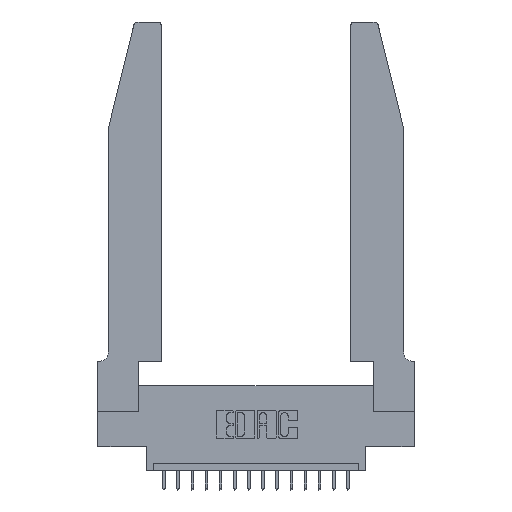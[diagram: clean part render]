
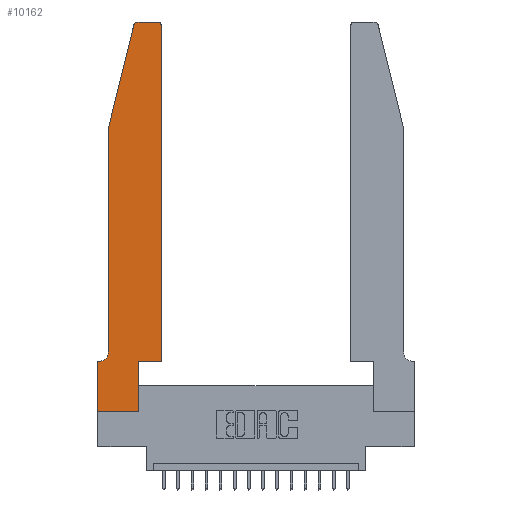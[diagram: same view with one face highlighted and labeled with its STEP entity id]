
A CAD part, top view. The second image highlights one B-rep face of the part: STEP entity #10162.
In plain terms, the highlighted planar face has unit normal (0, 0, 1).
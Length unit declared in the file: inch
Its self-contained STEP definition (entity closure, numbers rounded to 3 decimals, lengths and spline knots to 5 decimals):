
#179 = DIRECTION ( 'NONE',  ( 0., -1., 0. ) ) ;
#276 = EDGE_CURVE ( 'NONE', #15528, #753, #18520, .T. ) ;
#481 = DIRECTION ( 'NONE',  ( 1., 0., 0. ) ) ;
#716 = LINE ( 'NONE', #3756, #17238 ) ;
#753 = VERTEX_POINT ( 'NONE', #8095 ) ;
#1276 = CIRCLE ( 'NONE', #10348, 0.07 ) ;
#1418 = LINE ( 'NONE', #9024, #13395 ) ;
#1713 = VERTEX_POINT ( 'NONE', #18773 ) ;
#1873 = ORIENTED_EDGE ( 'NONE', *, *, #7005, .T. ) ;
#2048 = DIRECTION ( 'NONE',  ( 1., 0., 0. ) ) ;
#2084 = ORIENTED_EDGE ( 'NONE', *, *, #11575, .T. ) ;
#2132 = CARTESIAN_POINT ( 'NONE',  ( 0.4505, 0.35, 0.37 ) ) ;
#2269 = ORIENTED_EDGE ( 'NONE', *, *, #15552, .T. ) ;
#2403 = CARTESIAN_POINT ( 'NONE',  ( 0., 0.35, 0.37 ) ) ;
#2612 = EDGE_CURVE ( 'NONE', #7408, #15528, #11986, .T. ) ;
#2726 = LINE ( 'NONE', #2132, #7261 ) ;
#3155 = VECTOR ( 'NONE', #179, 39.37008 ) ;
#3355 = ORIENTED_EDGE ( 'NONE', *, *, #2612, .T. ) ;
#3377 = ORIENTED_EDGE ( 'NONE', *, *, #5155, .T. ) ;
#3412 = CARTESIAN_POINT ( 'NONE',  ( 0., 0., 0.37 ) ) ;
#3501 = VERTEX_POINT ( 'NONE', #7118 ) ;
#3566 = VECTOR ( 'NONE', #12857, 39.37008 ) ;
#3584 = PLANE ( 'NONE',  #14703 ) ;
#3756 = CARTESIAN_POINT ( 'NONE',  ( 0.0755, 2., 0.37 ) ) ;
#3758 = EDGE_CURVE ( 'NONE', #17499, #9092, #2726, .T. ) ;
#4745 = ORIENTED_EDGE ( 'NONE', *, *, #13297, .T. ) ;
#5133 = CARTESIAN_POINT ( 'NONE',  ( 0.2865, 0.35, 0.37 ) ) ;
#5155 = EDGE_CURVE ( 'NONE', #9092, #3501, #14441, .T. ) ;
#5293 = EDGE_CURVE ( 'NONE', #18282, #9228, #18702, .T. ) ;
#5518 = LINE ( 'NONE', #11480, #9516 ) ;
#5533 = CARTESIAN_POINT ( 'NONE',  ( 0.4505, 0.35, 0.37 ) ) ;
#5804 = CARTESIAN_POINT ( 'NONE',  ( 0.0755, 0.42, 0.37 ) ) ;
#6285 = AXIS2_PLACEMENT_3D ( 'NONE', #13538, #7651, #9419 ) ;
#6361 = CARTESIAN_POINT ( 'NONE',  ( 0.0055, 0.42, 0.37 ) ) ;
#6548 = DIRECTION ( 'NONE',  ( 0., 0., -1. ) ) ;
#6623 = CARTESIAN_POINT ( 'NONE',  ( 0.25487, 2.72718, 0.37 ) ) ;
#6675 = CARTESIAN_POINT ( 'NONE',  ( 0.0055, 0.35, 0.37 ) ) ;
#6748 = ORIENTED_EDGE ( 'NONE', *, *, #8304, .T. ) ;
#6881 = CARTESIAN_POINT ( 'NONE',  ( 0.0755, 2., 0.37 ) ) ;
#6970 = VECTOR ( 'NONE', #16101, 39.37008 ) ;
#7005 = EDGE_CURVE ( 'NONE', #10251, #7408, #1418, .T. ) ;
#7050 = DIRECTION ( 'NONE',  ( -1., 0., 0. ) ) ;
#7052 = VERTEX_POINT ( 'NONE', #5804 ) ;
#7118 = CARTESIAN_POINT ( 'NONE',  ( 0.4505, 2.72, 0.37 ) ) ;
#7261 = VECTOR ( 'NONE', #2048, 39.37008 ) ;
#7308 = CARTESIAN_POINT ( 'NONE',  ( 0.4505, 0.35, 0.37 ) ) ;
#7408 = VERTEX_POINT ( 'NONE', #13097 ) ;
#7572 = DIRECTION ( 'NONE',  ( 0., 0., 1. ) ) ;
#7651 = DIRECTION ( 'NONE',  ( 0., 0., 1. ) ) ;
#7834 = LINE ( 'NONE', #11001, #16626 ) ;
#8095 = CARTESIAN_POINT ( 'NONE',  ( 0.2865, 0., 0.37 ) ) ;
#8236 = ORIENTED_EDGE ( 'NONE', *, *, #13057, .T. ) ;
#8304 = EDGE_CURVE ( 'NONE', #7052, #10251, #1276, .T. ) ;
#8344 = VECTOR ( 'NONE', #481, 39.37008 ) ;
#9024 = CARTESIAN_POINT ( 'NONE',  ( 0.0755, 0.35, 0.37 ) ) ;
#9092 = VERTEX_POINT ( 'NONE', #5533 ) ;
#9107 = CARTESIAN_POINT ( 'NONE',  ( 0.0755, 2., 0.37 ) ) ;
#9228 = VERTEX_POINT ( 'NONE', #9107 ) ;
#9369 = CIRCLE ( 'NONE', #12194, 0.03 ) ;
#9419 = DIRECTION ( 'NONE',  ( 1., 0., 0. ) ) ;
#9516 = VECTOR ( 'NONE', #7050, 39.37008 ) ;
#9630 = DIRECTION ( 'NONE',  ( 0., 0., 1. ) ) ;
#9719 = DIRECTION ( 'NONE',  ( 0., -1., 0. ) ) ;
#9969 = VERTEX_POINT ( 'NONE', #18230 ) ;
#9974 = ORIENTED_EDGE ( 'NONE', *, *, #10007, .T. ) ;
#10007 = EDGE_CURVE ( 'NONE', #3501, #9969, #9369, .T. ) ;
#10162 = ADVANCED_FACE ( 'NONE', ( #15758 ), #3584, .T. ) ;
#10251 = VERTEX_POINT ( 'NONE', #6675 ) ;
#10348 = AXIS2_PLACEMENT_3D ( 'NONE', #6361, #6548, #10982 ) ;
#10982 = DIRECTION ( 'NONE',  ( -1., 0., 0. ) ) ;
#11001 = CARTESIAN_POINT ( 'NONE',  ( 0.2865, 0.35, 0.37 ) ) ;
#11196 = DIRECTION ( 'NONE',  ( 1., 0., 0. ) ) ;
#11480 = CARTESIAN_POINT ( 'NONE',  ( 0.2605, 2.75, 0.37 ) ) ;
#11575 = EDGE_CURVE ( 'NONE', #1713, #18282, #16592, .T. ) ;
#11986 = LINE ( 'NONE', #16273, #3155 ) ;
#12194 = AXIS2_PLACEMENT_3D ( 'NONE', #12276, #7572, #18043 ) ;
#12276 = CARTESIAN_POINT ( 'NONE',  ( 0.4205, 2.72, 0.37 ) ) ;
#12857 = DIRECTION ( 'NONE',  ( -0.239, -0.971, 0. ) ) ;
#13057 = EDGE_CURVE ( 'NONE', #753, #17499, #7834, .T. ) ;
#13097 = CARTESIAN_POINT ( 'NONE',  ( 0., 0.35, 0.37 ) ) ;
#13297 = EDGE_CURVE ( 'NONE', #9228, #7052, #716, .T. ) ;
#13395 = VECTOR ( 'NONE', #16243, 39.37008 ) ;
#13538 = CARTESIAN_POINT ( 'NONE',  ( 0.284, 2.72, 0.37 ) ) ;
#13722 = ORIENTED_EDGE ( 'NONE', *, *, #3758, .T. ) ;
#14441 = LINE ( 'NONE', #7308, #6970 ) ;
#14594 = CARTESIAN_POINT ( 'NONE',  ( 0., 0., 0.37 ) ) ;
#14703 = AXIS2_PLACEMENT_3D ( 'NONE', #2403, #9630, #11196 ) ;
#14927 = ORIENTED_EDGE ( 'NONE', *, *, #276, .T. ) ;
#15528 = VERTEX_POINT ( 'NONE', #14594 ) ;
#15552 = EDGE_CURVE ( 'NONE', #9969, #1713, #5518, .T. ) ;
#15758 = FACE_OUTER_BOUND ( 'NONE', #17296, .T. ) ;
#16101 = DIRECTION ( 'NONE',  ( 0., 1., 0. ) ) ;
#16243 = DIRECTION ( 'NONE',  ( -1., 0., 0. ) ) ;
#16273 = CARTESIAN_POINT ( 'NONE',  ( 0., 0., 0.37 ) ) ;
#16592 = CIRCLE ( 'NONE', #6285, 0.03 ) ;
#16626 = VECTOR ( 'NONE', #16841, 39.37008 ) ;
#16841 = DIRECTION ( 'NONE',  ( 0., 1., 0. ) ) ;
#17238 = VECTOR ( 'NONE', #9719, 39.37008 ) ;
#17296 = EDGE_LOOP ( 'NONE', ( #2269, #2084, #19132, #4745, #6748, #1873, #3355, #14927, #8236, #13722, #3377, #9974 ) ) ;
#17499 = VERTEX_POINT ( 'NONE', #5133 ) ;
#18043 = DIRECTION ( 'NONE',  ( 1., 0., 0. ) ) ;
#18230 = CARTESIAN_POINT ( 'NONE',  ( 0.4205, 2.75, 0.37 ) ) ;
#18282 = VERTEX_POINT ( 'NONE', #6623 ) ;
#18520 = LINE ( 'NONE', #3412, #8344 ) ;
#18702 = LINE ( 'NONE', #6881, #3566 ) ;
#18773 = CARTESIAN_POINT ( 'NONE',  ( 0.284, 2.75, 0.37 ) ) ;
#19132 = ORIENTED_EDGE ( 'NONE', *, *, #5293, .T. ) ;
